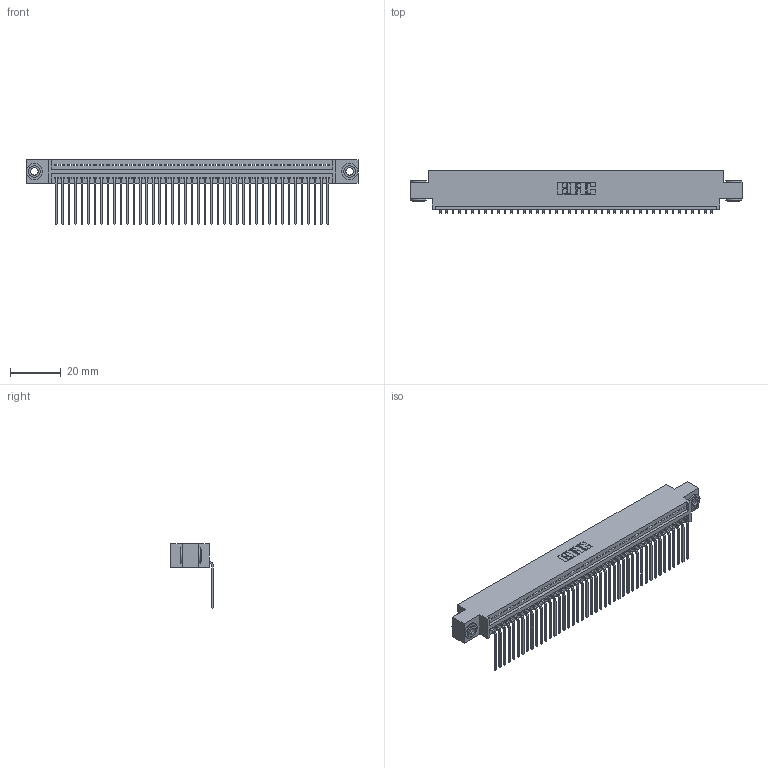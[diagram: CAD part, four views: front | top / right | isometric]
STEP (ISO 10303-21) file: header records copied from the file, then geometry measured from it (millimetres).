
FILE_DESCRIPTION (( 'STEP AP203' ), '1' );
FILE_NAME ('395-043-559-603.STEP', '2018-11-15T17:28:18', ( '' ), ( '' ), 'SwSTEP 2.0', 'SolidWorks 2016', '' );
FILE_SCHEMA (( 'CONFIG_CONTROL_DESIGN' ));
Length unit declared in the file: inch
Products named in the file (4): 345-250-002_345-250-002-102; 345 Part_0.170 Offset - 0.156 Dia-TH; 345-292-001_558 559 Tail - 1; 395-043-559-603
Assembly tree (46 placements, depth 2):
  395-043-559-603
    345 Part_0.170 Offset - 0.156 Dia-TH
    345-292-001_558 559 Tail - 1  x43
    345-250-002_345-250-002-102  x2
Bounding box: 130.43 x 16.75 x 25.53 mm (x, y, z)
Volume: 12445.7 mm3; surface area: 17735.7 mm2
Topology: 46 solids, 46 shells, 2748 faces, 8255 edges, 5442 vertices
Faces by surface type: plane 1900, cylinder 840, cone 8
Entity records: 33094 total; most frequent: CARTESIAN_POINT 5712, ORIENTED_EDGE 5682, DIRECTION 5017, EDGE_CURVE 2841, LINE 2513, VECTOR 2513, VERTEX_POINT 1890, AXIS2_PLACEMENT_3D 1252
